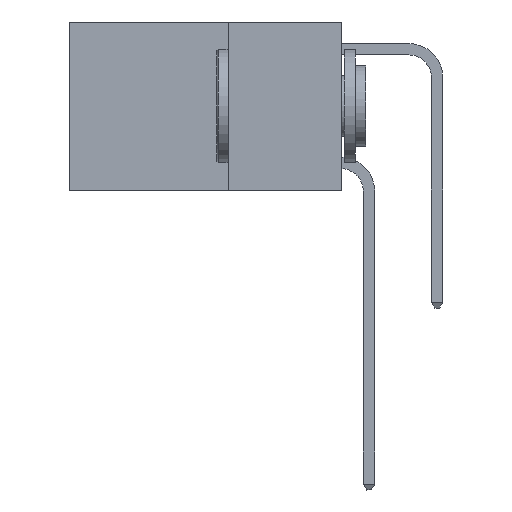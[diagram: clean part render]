
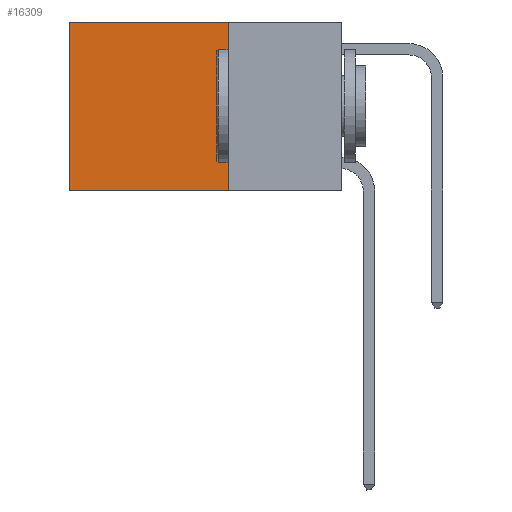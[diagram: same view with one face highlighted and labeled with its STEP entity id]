
A CAD part, left-side view. The second image highlights one B-rep face of the part: STEP entity #16309.
In plain terms, the highlighted planar face has unit normal (-1, 0, 0).
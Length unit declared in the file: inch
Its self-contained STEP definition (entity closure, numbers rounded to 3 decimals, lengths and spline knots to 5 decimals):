
#726 = EDGE_CURVE ( 'NONE', #10005, #22471, #17520, .T. ) ;
#1832 = ORIENTED_EDGE ( 'NONE', *, *, #16390, .F. ) ;
#1905 = VECTOR ( 'NONE', #15638, 39.37008 ) ;
#2379 = PLANE ( 'NONE',  #23332 ) ;
#2570 = EDGE_CURVE ( 'NONE', #16754, #9703, #2730, .T. ) ;
#2730 = LINE ( 'NONE', #18045, #22755 ) ;
#3800 = VECTOR ( 'NONE', #12420, 39.37008 ) ;
#4007 = DIRECTION ( 'NONE',  ( 1., 0., 0. ) ) ;
#4221 = CARTESIAN_POINT ( 'NONE',  ( 0.2625, 0.25, 0. ) ) ;
#4254 = CARTESIAN_POINT ( 'NONE',  ( 0.2625, 0.25, 0. ) ) ;
#4733 = ORIENTED_EDGE ( 'NONE', *, *, #726, .F. ) ;
#5262 = ORIENTED_EDGE ( 'NONE', *, *, #2570, .T. ) ;
#5434 = CARTESIAN_POINT ( 'NONE',  ( 0.2625, 0.6, 0. ) ) ;
#6129 = CARTESIAN_POINT ( 'NONE',  ( 0.2625, 0.25, 0. ) ) ;
#7034 = CARTESIAN_POINT ( 'NONE',  ( 0.2625, 0.6, -0.37 ) ) ;
#7058 = CARTESIAN_POINT ( 'NONE',  ( 0.2625, 0.6, 0. ) ) ;
#9703 = VERTEX_POINT ( 'NONE', #5434 ) ;
#9989 = DIRECTION ( 'NONE',  ( 0., 0., -1. ) ) ;
#10005 = VERTEX_POINT ( 'NONE', #22049 ) ;
#10341 = DIRECTION ( 'NONE',  ( 0., 1., 0. ) ) ;
#11547 = CARTESIAN_POINT ( 'NONE',  ( 0.2625, 0.25, -0.37 ) ) ;
#12420 = DIRECTION ( 'NONE',  ( 0., 0., -1. ) ) ;
#13870 = EDGE_CURVE ( 'NONE', #9703, #22471, #20138, .T. ) ;
#15638 = DIRECTION ( 'NONE',  ( 0., 1., 0. ) ) ;
#15844 = LINE ( 'NONE', #4254, #22937 ) ;
#16030 = ORIENTED_EDGE ( 'NONE', *, *, #13870, .T. ) ;
#16309 = ADVANCED_FACE ( 'NONE', ( #23319 ), #2379, .F. ) ;
#16390 = EDGE_CURVE ( 'NONE', #16754, #10005, #15844, .T. ) ;
#16754 = VERTEX_POINT ( 'NONE', #4221 ) ;
#17520 = LINE ( 'NONE', #11547, #1905 ) ;
#18045 = CARTESIAN_POINT ( 'NONE',  ( 0.2625, 0.25, 0. ) ) ;
#19332 = DIRECTION ( 'NONE',  ( 0., 0., -1. ) ) ;
#19453 = EDGE_LOOP ( 'NONE', ( #16030, #4733, #1832, #5262 ) ) ;
#20138 = LINE ( 'NONE', #7058, #3800 ) ;
#22049 = CARTESIAN_POINT ( 'NONE',  ( 0.2625, 0.25, -0.37 ) ) ;
#22471 = VERTEX_POINT ( 'NONE', #7034 ) ;
#22755 = VECTOR ( 'NONE', #10341, 39.37008 ) ;
#22937 = VECTOR ( 'NONE', #19332, 39.37008 ) ;
#23319 = FACE_OUTER_BOUND ( 'NONE', #19453, .T. ) ;
#23332 = AXIS2_PLACEMENT_3D ( 'NONE', #6129, #4007, #9989 ) ;
